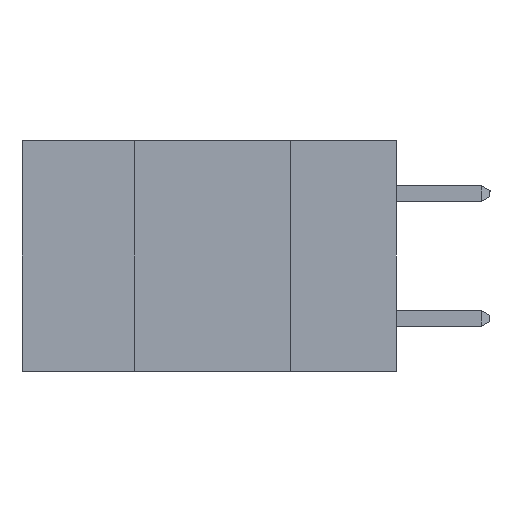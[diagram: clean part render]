
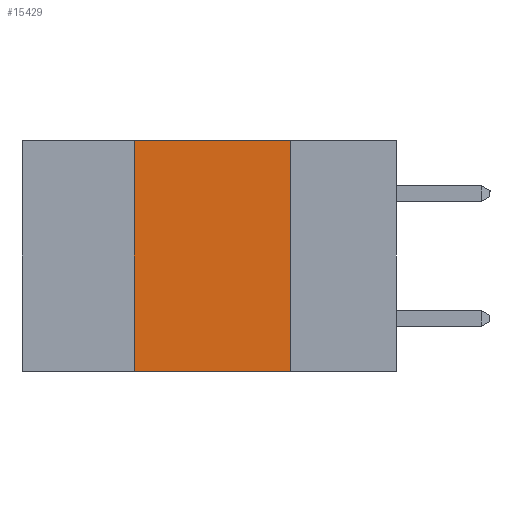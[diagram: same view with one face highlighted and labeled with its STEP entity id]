
A CAD part, left-side view. The second image highlights one B-rep face of the part: STEP entity #15429.
In plain terms, the highlighted planar face has unit normal (-1, 0, 0).
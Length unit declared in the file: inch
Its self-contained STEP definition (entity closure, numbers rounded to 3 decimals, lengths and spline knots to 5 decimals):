
#64 = PLANE ( 'NONE',  #12895 ) ;
#1943 = CARTESIAN_POINT ( 'NONE',  ( 0., 0.17, -0.37 ) ) ;
#3607 = CARTESIAN_POINT ( 'NONE',  ( 0., 0.17, 0. ) ) ;
#3948 = VERTEX_POINT ( 'NONE', #11254 ) ;
#5089 = DIRECTION ( 'NONE',  ( 0., -1., 0. ) ) ;
#5556 = ORIENTED_EDGE ( 'NONE', *, *, #12105, .F. ) ;
#5588 = CARTESIAN_POINT ( 'NONE',  ( 0., 0.17, -0.37 ) ) ;
#5848 = EDGE_CURVE ( 'NONE', #11402, #6878, #16466, .T. ) ;
#6878 = VERTEX_POINT ( 'NONE', #5588 ) ;
#7519 = CARTESIAN_POINT ( 'NONE',  ( 0., 0.42, -0.37 ) ) ;
#8441 = VECTOR ( 'NONE', #12532, 39.37008 ) ;
#9120 = DIRECTION ( 'NONE',  ( 0., 0., -1. ) ) ;
#9551 = VECTOR ( 'NONE', #5089, 39.37008 ) ;
#9985 = LINE ( 'NONE', #11305, #17357 ) ;
#11254 = CARTESIAN_POINT ( 'NONE',  ( 0., 0.42, 0. ) ) ;
#11305 = CARTESIAN_POINT ( 'NONE',  ( 0., 0.42, -0.37 ) ) ;
#11402 = VERTEX_POINT ( 'NONE', #7519 ) ;
#11458 = CARTESIAN_POINT ( 'NONE',  ( 0., 0.6, 0. ) ) ;
#12105 = EDGE_CURVE ( 'NONE', #3948, #16078, #12723, .T. ) ;
#12532 = DIRECTION ( 'NONE',  ( 0., -1., 0. ) ) ;
#12723 = LINE ( 'NONE', #15451, #8441 ) ;
#12727 = VECTOR ( 'NONE', #9120, 39.37008 ) ;
#12895 = AXIS2_PLACEMENT_3D ( 'NONE', #11458, #17258, #14352 ) ;
#14104 = DIRECTION ( 'NONE',  ( 0., 0., 1. ) ) ;
#14352 = DIRECTION ( 'NONE',  ( 0., 0., -1. ) ) ;
#14459 = ORIENTED_EDGE ( 'NONE', *, *, #17404, .F. ) ;
#14731 = LINE ( 'NONE', #1943, #12727 ) ;
#14785 = EDGE_CURVE ( 'NONE', #11402, #3948, #9985, .T. ) ;
#15429 = ADVANCED_FACE ( 'NONE', ( #16043 ), #64, .F. ) ;
#15451 = CARTESIAN_POINT ( 'NONE',  ( 0., 0.6, 0. ) ) ;
#16043 = FACE_OUTER_BOUND ( 'NONE', #18067, .T. ) ;
#16078 = VERTEX_POINT ( 'NONE', #3607 ) ;
#16134 = ORIENTED_EDGE ( 'NONE', *, *, #14785, .F. ) ;
#16466 = LINE ( 'NONE', #18060, #9551 ) ;
#17027 = ORIENTED_EDGE ( 'NONE', *, *, #5848, .T. ) ;
#17258 = DIRECTION ( 'NONE',  ( 1., 0., 0. ) ) ;
#17357 = VECTOR ( 'NONE', #14104, 39.37008 ) ;
#17404 = EDGE_CURVE ( 'NONE', #16078, #6878, #14731, .T. ) ;
#18060 = CARTESIAN_POINT ( 'NONE',  ( 0., 0.6, -0.37 ) ) ;
#18067 = EDGE_LOOP ( 'NONE', ( #14459, #5556, #16134, #17027 ) ) ;
